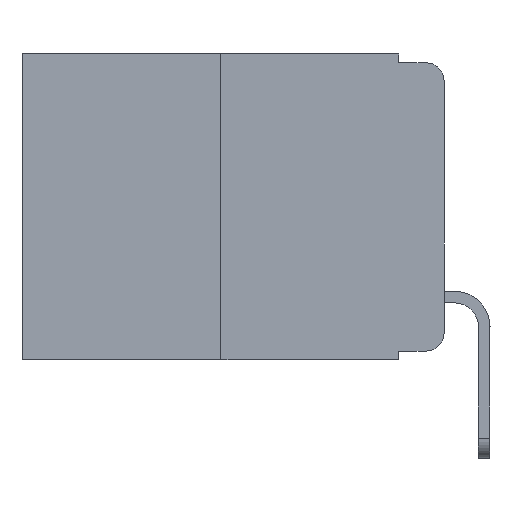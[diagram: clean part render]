
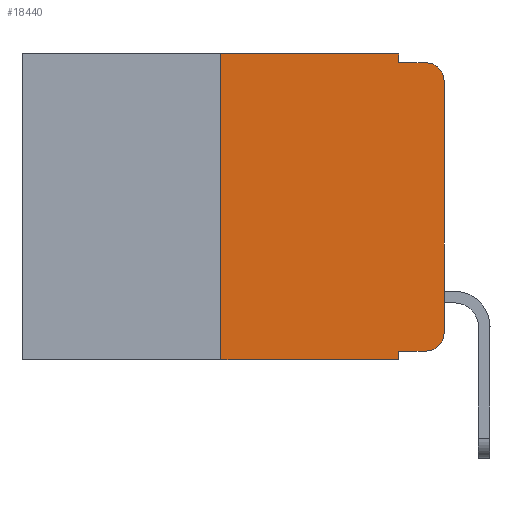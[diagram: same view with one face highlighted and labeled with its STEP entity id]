
A CAD part, left-side view. The second image highlights one B-rep face of the part: STEP entity #18440.
In plain terms, the highlighted planar face has unit normal (-1, 0, 0).
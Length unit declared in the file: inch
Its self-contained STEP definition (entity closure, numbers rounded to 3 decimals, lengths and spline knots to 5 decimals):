
#583 = CARTESIAN_POINT ( 'NONE',  ( 0., 0.02, -0.313 ) ) ;
#606 = PLANE ( 'NONE',  #6921 ) ;
#617 = VECTOR ( 'NONE', #4611, 39.37008 ) ;
#867 = ORIENTED_EDGE ( 'NONE', *, *, #13407, .F. ) ;
#1953 = ORIENTED_EDGE ( 'NONE', *, *, #15719, .T. ) ;
#2324 = DIRECTION ( 'NONE',  ( -1., 0., 0. ) ) ;
#2343 = VERTEX_POINT ( 'NONE', #4363 ) ;
#2748 = VERTEX_POINT ( 'NONE', #15610 ) ;
#2900 = ORIENTED_EDGE ( 'NONE', *, *, #7794, .F. ) ;
#3311 = LINE ( 'NONE', #11744, #11349 ) ;
#3323 = CARTESIAN_POINT ( 'NONE',  ( 0., 0.051, 0. ) ) ;
#3442 = DIRECTION ( 'NONE',  ( 0., -1., 0. ) ) ;
#3461 = VECTOR ( 'NONE', #19648, 39.37008 ) ;
#3551 = CIRCLE ( 'NONE', #6287, 0.02 ) ;
#3762 = DIRECTION ( 'NONE',  ( 0., 0., -1. ) ) ;
#4160 = CIRCLE ( 'NONE', #12465, 0.02 ) ;
#4197 = CARTESIAN_POINT ( 'NONE',  ( 0., 0.02, -0.01 ) ) ;
#4363 = CARTESIAN_POINT ( 'NONE',  ( 0., 0.25, 0. ) ) ;
#4394 = CARTESIAN_POINT ( 'NONE',  ( 0., 0.25, -0.343 ) ) ;
#4499 = DIRECTION ( 'NONE',  ( 0., 0., -1. ) ) ;
#4611 = DIRECTION ( 'NONE',  ( 0., 0., 1. ) ) ;
#4791 = CARTESIAN_POINT ( 'NONE',  ( 0., 0.02, -0.03 ) ) ;
#5139 = VECTOR ( 'NONE', #3442, 39.37008 ) ;
#5280 = FACE_OUTER_BOUND ( 'NONE', #9462, .T. ) ;
#5553 = DIRECTION ( 'NONE',  ( 0., -1., 0. ) ) ;
#5691 = VERTEX_POINT ( 'NONE', #13446 ) ;
#5736 = ORIENTED_EDGE ( 'NONE', *, *, #16519, .F. ) ;
#6287 = AXIS2_PLACEMENT_3D ( 'NONE', #583, #2324, #6856 ) ;
#6809 = VECTOR ( 'NONE', #10567, 39.37008 ) ;
#6856 = DIRECTION ( 'NONE',  ( 0., 0., -1. ) ) ;
#6921 = AXIS2_PLACEMENT_3D ( 'NONE', #10545, #16883, #3762 ) ;
#7119 = CARTESIAN_POINT ( 'NONE',  ( 0., 0.051, 0. ) ) ;
#7651 = EDGE_CURVE ( 'NONE', #9418, #8518, #13220, .T. ) ;
#7703 = DIRECTION ( 'NONE',  ( -1., 0., 0. ) ) ;
#7794 = EDGE_CURVE ( 'NONE', #9796, #2748, #17243, .T. ) ;
#8090 = EDGE_CURVE ( 'NONE', #12622, #5691, #16460, .T. ) ;
#8352 = VERTEX_POINT ( 'NONE', #19454 ) ;
#8518 = VERTEX_POINT ( 'NONE', #8649 ) ;
#8593 = ORIENTED_EDGE ( 'NONE', *, *, #8090, .T. ) ;
#8649 = CARTESIAN_POINT ( 'NONE',  ( 0., 0., -0.03 ) ) ;
#8936 = CARTESIAN_POINT ( 'NONE',  ( 0., 0.473, -0.343 ) ) ;
#9204 = LINE ( 'NONE', #12268, #12561 ) ;
#9231 = CARTESIAN_POINT ( 'NONE',  ( 0., 0.051, 0. ) ) ;
#9418 = VERTEX_POINT ( 'NONE', #9806 ) ;
#9462 = EDGE_LOOP ( 'NONE', ( #17877, #14291, #867, #2900, #5736, #16210, #1953, #17179, #8593, #14353 ) ) ;
#9551 = LINE ( 'NONE', #9231, #19599 ) ;
#9796 = VERTEX_POINT ( 'NONE', #3323 ) ;
#9806 = CARTESIAN_POINT ( 'NONE',  ( 0., 0., -0.313 ) ) ;
#10037 = CARTESIAN_POINT ( 'NONE',  ( 0., 0., 0. ) ) ;
#10545 = CARTESIAN_POINT ( 'NONE',  ( 0., 0.473, 0. ) ) ;
#10567 = DIRECTION ( 'NONE',  ( 0., -1., 0. ) ) ;
#10678 = EDGE_CURVE ( 'NONE', #13059, #2343, #14749, .T. ) ;
#11349 = VECTOR ( 'NONE', #11960, 39.37008 ) ;
#11744 = CARTESIAN_POINT ( 'NONE',  ( 0., 0.473, 0. ) ) ;
#11960 = DIRECTION ( 'NONE',  ( 0., -1., 0. ) ) ;
#12268 = CARTESIAN_POINT ( 'NONE',  ( 0., 0.051, -0.01 ) ) ;
#12322 = CARTESIAN_POINT ( 'NONE',  ( 0., 0.051, -0.333 ) ) ;
#12465 = AXIS2_PLACEMENT_3D ( 'NONE', #4791, #7703, #19349 ) ;
#12561 = VECTOR ( 'NONE', #5553, 39.37008 ) ;
#12622 = VERTEX_POINT ( 'NONE', #12322 ) ;
#13059 = VERTEX_POINT ( 'NONE', #4394 ) ;
#13220 = LINE ( 'NONE', #10037, #617 ) ;
#13400 = CARTESIAN_POINT ( 'NONE',  ( 0., 0.051, -0.333 ) ) ;
#13407 = EDGE_CURVE ( 'NONE', #2748, #19831, #9204, .T. ) ;
#13446 = CARTESIAN_POINT ( 'NONE',  ( 0., 0.02, -0.333 ) ) ;
#13641 = DIRECTION ( 'NONE',  ( 0., 0., -1. ) ) ;
#13848 = LINE ( 'NONE', #8936, #6809 ) ;
#14291 = ORIENTED_EDGE ( 'NONE', *, *, #18075, .T. ) ;
#14353 = ORIENTED_EDGE ( 'NONE', *, *, #20062, .T. ) ;
#14749 = LINE ( 'NONE', #21278, #3461 ) ;
#15069 = EDGE_CURVE ( 'NONE', #12622, #8352, #9551, .T. ) ;
#15610 = CARTESIAN_POINT ( 'NONE',  ( 0., 0.051, -0.01 ) ) ;
#15719 = EDGE_CURVE ( 'NONE', #13059, #8352, #13848, .T. ) ;
#16210 = ORIENTED_EDGE ( 'NONE', *, *, #10678, .F. ) ;
#16460 = LINE ( 'NONE', #13400, #5139 ) ;
#16519 = EDGE_CURVE ( 'NONE', #2343, #9796, #3311, .T. ) ;
#16883 = DIRECTION ( 'NONE',  ( 1., 0., 0. ) ) ;
#17179 = ORIENTED_EDGE ( 'NONE', *, *, #15069, .F. ) ;
#17243 = LINE ( 'NONE', #7119, #17966 ) ;
#17877 = ORIENTED_EDGE ( 'NONE', *, *, #7651, .T. ) ;
#17966 = VECTOR ( 'NONE', #13641, 39.37008 ) ;
#18075 = EDGE_CURVE ( 'NONE', #8518, #19831, #4160, .T. ) ;
#18440 = ADVANCED_FACE ( 'NONE', ( #5280 ), #606, .F. ) ;
#19349 = DIRECTION ( 'NONE',  ( 0., 0., -1. ) ) ;
#19454 = CARTESIAN_POINT ( 'NONE',  ( 0., 0.051, -0.343 ) ) ;
#19599 = VECTOR ( 'NONE', #4499, 39.37008 ) ;
#19648 = DIRECTION ( 'NONE',  ( 0., 0., 1. ) ) ;
#19831 = VERTEX_POINT ( 'NONE', #4197 ) ;
#20062 = EDGE_CURVE ( 'NONE', #5691, #9418, #3551, .T. ) ;
#21278 = CARTESIAN_POINT ( 'NONE',  ( 0., 0.25, 0. ) ) ;
